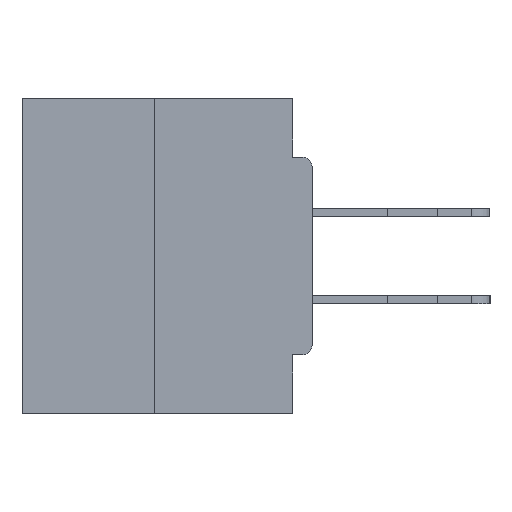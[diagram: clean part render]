
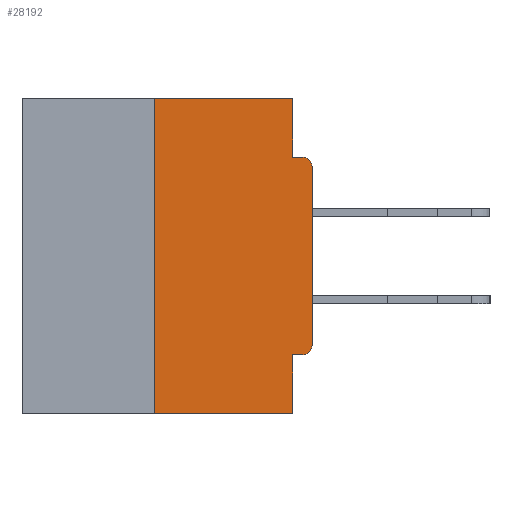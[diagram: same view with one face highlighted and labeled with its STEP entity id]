
A CAD part, left-side view. The second image highlights one B-rep face of the part: STEP entity #28192.
In plain terms, the highlighted planar face has unit normal (-1, 0, 0).
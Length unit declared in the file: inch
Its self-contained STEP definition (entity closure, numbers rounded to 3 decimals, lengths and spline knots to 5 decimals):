
#1191 = CARTESIAN_POINT ( 'NONE',  ( 0., 0.031, -0.5 ) ) ;
#2013 = VERTEX_POINT ( 'NONE', #25610 ) ;
#2287 = LINE ( 'NONE', #13834, #14622 ) ;
#2506 = CARTESIAN_POINT ( 'NONE',  ( 0., 0., 0. ) ) ;
#2911 = VERTEX_POINT ( 'NONE', #27404 ) ;
#2962 = AXIS2_PLACEMENT_3D ( 'NONE', #35228, #13373, #27477 ) ;
#3741 = VERTEX_POINT ( 'NONE', #31079 ) ;
#4156 = VECTOR ( 'NONE', #24089, 39.37008 ) ;
#4174 = EDGE_LOOP ( 'NONE', ( #9035, #17504, #20982, #7072, #6339, #31811, #25311, #10875, #28143, #25398 ) ) ;
#4368 = CIRCLE ( 'NONE', #5542, 0.015 ) ;
#5542 = AXIS2_PLACEMENT_3D ( 'NONE', #12405, #25786, #25911 ) ;
#5646 = DIRECTION ( 'NONE',  ( 0., -1., 0. ) ) ;
#5877 = EDGE_CURVE ( 'NONE', #3741, #22106, #2287, .T. ) ;
#6339 = ORIENTED_EDGE ( 'NONE', *, *, #14842, .F. ) ;
#6564 = CARTESIAN_POINT ( 'NONE',  ( 0., 0., -0.4065 ) ) ;
#6572 = EDGE_CURVE ( 'NONE', #2013, #22850, #27817, .T. ) ;
#6741 = EDGE_CURVE ( 'NONE', #23432, #23444, #4368, .T. ) ;
#6966 = DIRECTION ( 'NONE',  ( 0., -1., 0. ) ) ;
#7072 = ORIENTED_EDGE ( 'NONE', *, *, #5877, .F. ) ;
#7414 = VERTEX_POINT ( 'NONE', #34123 ) ;
#8014 = PLANE ( 'NONE',  #2962 ) ;
#8349 = CARTESIAN_POINT ( 'NONE',  ( 0., 0.031, 0. ) ) ;
#8501 = VECTOR ( 'NONE', #25656, 39.37008 ) ;
#8536 = LINE ( 'NONE', #23305, #16198 ) ;
#8585 = LINE ( 'NONE', #31333, #14995 ) ;
#9035 = ORIENTED_EDGE ( 'NONE', *, *, #12531, .F. ) ;
#10741 = CIRCLE ( 'NONE', #25071, 0.015 ) ;
#10875 = ORIENTED_EDGE ( 'NONE', *, *, #12155, .T. ) ;
#11743 = VECTOR ( 'NONE', #5646, 39.37008 ) ;
#12155 = EDGE_CURVE ( 'NONE', #2911, #25415, #10741, .T. ) ;
#12405 = CARTESIAN_POINT ( 'NONE',  ( 0., 0.015, -0.3915 ) ) ;
#12531 = EDGE_CURVE ( 'NONE', #16449, #2013, #8585, .T. ) ;
#12873 = CARTESIAN_POINT ( 'NONE',  ( 0., 0., -0.3915 ) ) ;
#13373 = DIRECTION ( 'NONE',  ( 1., 0., 0. ) ) ;
#13391 = DIRECTION ( 'NONE',  ( -1., 0., 0. ) ) ;
#13834 = CARTESIAN_POINT ( 'NONE',  ( 0., 0.031, -0.5 ) ) ;
#14324 = EDGE_CURVE ( 'NONE', #7414, #22106, #8536, .T. ) ;
#14622 = VECTOR ( 'NONE', #16560, 39.37008 ) ;
#14842 = EDGE_CURVE ( 'NONE', #23432, #3741, #14922, .T. ) ;
#14922 = LINE ( 'NONE', #6564, #8501 ) ;
#14995 = VECTOR ( 'NONE', #6966, 39.37008 ) ;
#16198 = VECTOR ( 'NONE', #31813, 39.37008 ) ;
#16431 = FACE_OUTER_BOUND ( 'NONE', #4174, .T. ) ;
#16449 = VERTEX_POINT ( 'NONE', #31281 ) ;
#16547 = LINE ( 'NONE', #19373, #31569 ) ;
#16560 = DIRECTION ( 'NONE',  ( 0., 0., -1. ) ) ;
#17504 = ORIENTED_EDGE ( 'NONE', *, *, #26500, .F. ) ;
#19373 = CARTESIAN_POINT ( 'NONE',  ( 0., 0.25, 0. ) ) ;
#20982 = ORIENTED_EDGE ( 'NONE', *, *, #14324, .T. ) ;
#22078 = DIRECTION ( 'NONE',  ( 0., 0., -1. ) ) ;
#22106 = VERTEX_POINT ( 'NONE', #1191 ) ;
#22850 = VERTEX_POINT ( 'NONE', #29071 ) ;
#23305 = CARTESIAN_POINT ( 'NONE',  ( 0., 0.46, -0.5 ) ) ;
#23432 = VERTEX_POINT ( 'NONE', #29496 ) ;
#23444 = VERTEX_POINT ( 'NONE', #12873 ) ;
#24089 = DIRECTION ( 'NONE',  ( 0., 0., 1. ) ) ;
#25071 = AXIS2_PLACEMENT_3D ( 'NONE', #32773, #13391, #32887 ) ;
#25241 = DIRECTION ( 'NONE',  ( 0., 0., 1. ) ) ;
#25311 = ORIENTED_EDGE ( 'NONE', *, *, #27643, .T. ) ;
#25398 = ORIENTED_EDGE ( 'NONE', *, *, #6572, .F. ) ;
#25415 = VERTEX_POINT ( 'NONE', #32306 ) ;
#25610 = CARTESIAN_POINT ( 'NONE',  ( 0., 0.031, 0. ) ) ;
#25656 = DIRECTION ( 'NONE',  ( 0., 1., 0. ) ) ;
#25786 = DIRECTION ( 'NONE',  ( -1., 0., 0. ) ) ;
#25911 = DIRECTION ( 'NONE',  ( 0., 0., -1. ) ) ;
#26500 = EDGE_CURVE ( 'NONE', #7414, #16449, #16547, .T. ) ;
#27404 = CARTESIAN_POINT ( 'NONE',  ( 0., 0., -0.1085 ) ) ;
#27477 = DIRECTION ( 'NONE',  ( 0., 0., -1. ) ) ;
#27553 = LINE ( 'NONE', #32641, #11743 ) ;
#27643 = EDGE_CURVE ( 'NONE', #23444, #2911, #34881, .T. ) ;
#27817 = LINE ( 'NONE', #8349, #34683 ) ;
#28143 = ORIENTED_EDGE ( 'NONE', *, *, #28266, .F. ) ;
#28192 = ADVANCED_FACE ( 'NONE', ( #16431 ), #8014, .F. ) ;
#28266 = EDGE_CURVE ( 'NONE', #22850, #25415, #27553, .T. ) ;
#29071 = CARTESIAN_POINT ( 'NONE',  ( 0., 0.031, -0.0935 ) ) ;
#29496 = CARTESIAN_POINT ( 'NONE',  ( 0., 0.015, -0.4065 ) ) ;
#31079 = CARTESIAN_POINT ( 'NONE',  ( 0., 0.031, -0.4065 ) ) ;
#31281 = CARTESIAN_POINT ( 'NONE',  ( 0., 0.25, 0. ) ) ;
#31333 = CARTESIAN_POINT ( 'NONE',  ( 0., 0.46, 0. ) ) ;
#31569 = VECTOR ( 'NONE', #25241, 39.37008 ) ;
#31811 = ORIENTED_EDGE ( 'NONE', *, *, #6741, .T. ) ;
#31813 = DIRECTION ( 'NONE',  ( 0., -1., 0. ) ) ;
#32306 = CARTESIAN_POINT ( 'NONE',  ( 0., 0.015, -0.0935 ) ) ;
#32641 = CARTESIAN_POINT ( 'NONE',  ( 0., 0., -0.0935 ) ) ;
#32773 = CARTESIAN_POINT ( 'NONE',  ( 0., 0.015, -0.1085 ) ) ;
#32887 = DIRECTION ( 'NONE',  ( 0., 0., -1. ) ) ;
#34123 = CARTESIAN_POINT ( 'NONE',  ( 0., 0.25, -0.5 ) ) ;
#34683 = VECTOR ( 'NONE', #22078, 39.37008 ) ;
#34881 = LINE ( 'NONE', #2506, #4156 ) ;
#35228 = CARTESIAN_POINT ( 'NONE',  ( 0., 0.46, 0. ) ) ;
